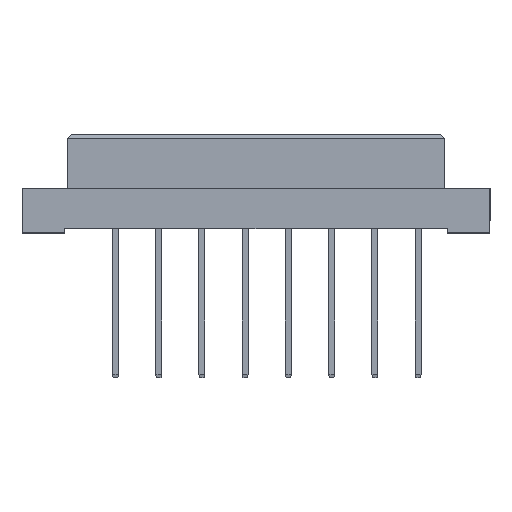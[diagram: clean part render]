
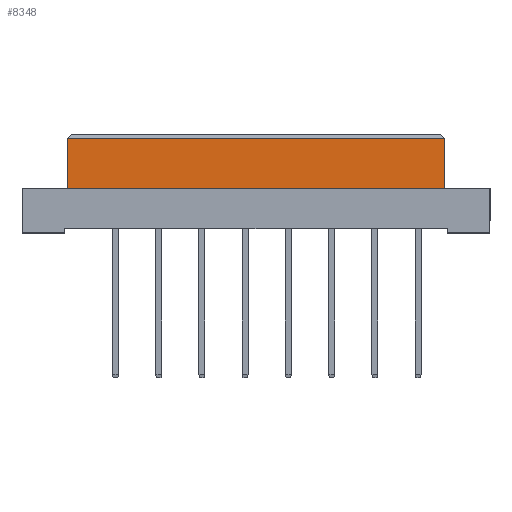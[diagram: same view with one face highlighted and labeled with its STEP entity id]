
A CAD part, top view. The second image highlights one B-rep face of the part: STEP entity #8348.
In plain terms, the highlighted planar face has unit normal (0, 0, 1).
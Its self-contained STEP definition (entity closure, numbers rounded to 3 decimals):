
#564 = DIRECTION ( 'NONE',  ( -1., 0., 0. ) ) ;
#682 = ORIENTED_EDGE ( 'NONE', *, *, #18385, .T. ) ;
#1159 = CARTESIAN_POINT ( 'NONE',  ( -22.2, -0.5, 4.25 ) ) ;
#2504 = CARTESIAN_POINT ( 'NONE',  ( 22.2, -6.4, 4.25 ) ) ;
#2726 = EDGE_CURVE ( 'NONE', #11753, #15855, #3479, .T. ) ;
#3479 = LINE ( 'NONE', #11402, #13076 ) ;
#5179 = ORIENTED_EDGE ( 'NONE', *, *, #19910, .F. ) ;
#5627 = LINE ( 'NONE', #18020, #8917 ) ;
#5874 = VERTEX_POINT ( 'NONE', #16811 ) ;
#6459 = VECTOR ( 'NONE', #564, 1000. ) ;
#7262 = DIRECTION ( 'NONE',  ( 0., 0., 1. ) ) ;
#7372 = CARTESIAN_POINT ( 'NONE',  ( 22.2, -6.4, 4.25 ) ) ;
#7592 = VECTOR ( 'NONE', #14990, 1000. ) ;
#8348 = ADVANCED_FACE ( 'NONE', ( #19671 ), #8700, .T. ) ;
#8700 = PLANE ( 'NONE',  #9355 ) ;
#8917 = VECTOR ( 'NONE', #18215, 1000. ) ;
#9245 = VERTEX_POINT ( 'NONE', #1159 ) ;
#9355 = AXIS2_PLACEMENT_3D ( 'NONE', #10133, #7262, #19463 ) ;
#10133 = CARTESIAN_POINT ( 'NONE',  ( 22.2, -6.4, 4.25 ) ) ;
#10235 = CARTESIAN_POINT ( 'NONE',  ( 22.2, -0.5, 4.25 ) ) ;
#10881 = ORIENTED_EDGE ( 'NONE', *, *, #2726, .T. ) ;
#11296 = EDGE_LOOP ( 'NONE', ( #10881, #16297, #5179, #682 ) ) ;
#11402 = CARTESIAN_POINT ( 'NONE',  ( 22.2, -6.4, 4.25 ) ) ;
#11660 = LINE ( 'NONE', #17992, #6459 ) ;
#11753 = VERTEX_POINT ( 'NONE', #2504 ) ;
#13076 = VECTOR ( 'NONE', #14372, 1000. ) ;
#14372 = DIRECTION ( 'NONE',  ( 0., 1., 0. ) ) ;
#14990 = DIRECTION ( 'NONE',  ( 1., 0., 0. ) ) ;
#15855 = VERTEX_POINT ( 'NONE', #10235 ) ;
#16297 = ORIENTED_EDGE ( 'NONE', *, *, #17465, .T. ) ;
#16811 = CARTESIAN_POINT ( 'NONE',  ( -22.2, -6.4, 4.25 ) ) ;
#17465 = EDGE_CURVE ( 'NONE', #15855, #9245, #11660, .T. ) ;
#17992 = CARTESIAN_POINT ( 'NONE',  ( -22.2, -0.5, 4.25 ) ) ;
#18020 = CARTESIAN_POINT ( 'NONE',  ( -22.2, -6.4, 4.25 ) ) ;
#18215 = DIRECTION ( 'NONE',  ( 0., 1., 0. ) ) ;
#18385 = EDGE_CURVE ( 'NONE', #5874, #11753, #19691, .T. ) ;
#19463 = DIRECTION ( 'NONE',  ( 1., 0., 0. ) ) ;
#19671 = FACE_OUTER_BOUND ( 'NONE', #11296, .T. ) ;
#19691 = LINE ( 'NONE', #7372, #7592 ) ;
#19910 = EDGE_CURVE ( 'NONE', #5874, #9245, #5627, .T. ) ;
